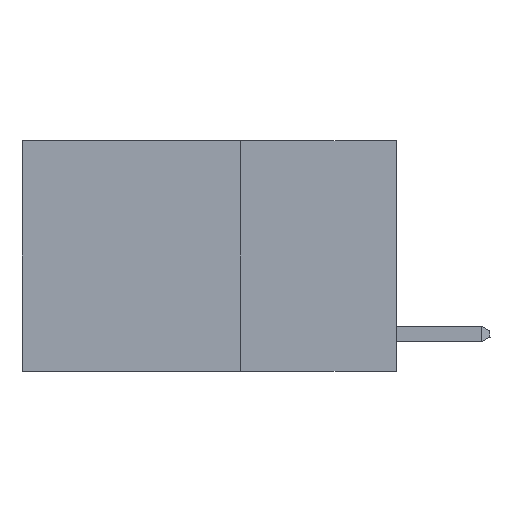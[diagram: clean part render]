
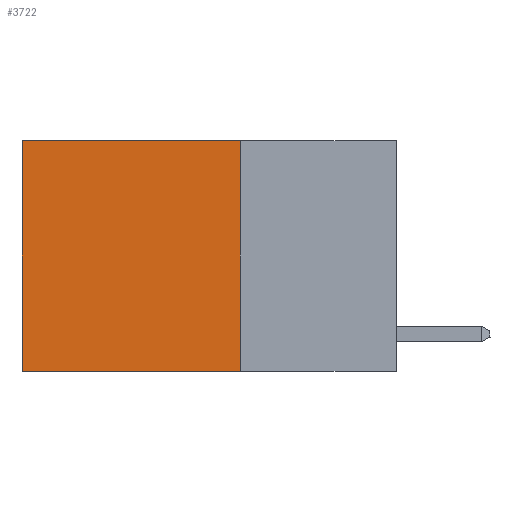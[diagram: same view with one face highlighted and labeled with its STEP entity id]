
A CAD part, left-side view. The second image highlights one B-rep face of the part: STEP entity #3722.
In plain terms, the highlighted planar face has unit normal (-1, 0, 0).
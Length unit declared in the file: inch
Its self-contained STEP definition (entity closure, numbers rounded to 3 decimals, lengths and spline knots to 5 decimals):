
#105 = CARTESIAN_POINT ( 'NONE',  ( 0.2625, 0.6, -0.37 ) ) ;
#321 = CARTESIAN_POINT ( 'NONE',  ( 0.2625, 0.25, -0.37 ) ) ;
#519 = CARTESIAN_POINT ( 'NONE',  ( 0.2625, 0.25, 0. ) ) ;
#686 = DIRECTION ( 'NONE',  ( 0., 0., -1. ) ) ;
#990 = CARTESIAN_POINT ( 'NONE',  ( 0.2625, 0.25, 0. ) ) ;
#2225 = VECTOR ( 'NONE', #8010, 39.37008 ) ;
#2432 = ORIENTED_EDGE ( 'NONE', *, *, #14930, .T. ) ;
#2452 = VERTEX_POINT ( 'NONE', #105 ) ;
#2832 = LINE ( 'NONE', #20732, #2225 ) ;
#3722 = ADVANCED_FACE ( 'NONE', ( #22056 ), #22580, .F. ) ;
#4073 = EDGE_LOOP ( 'NONE', ( #18941, #13759, #9284, #2432 ) ) ;
#4155 = DIRECTION ( 'NONE',  ( 0., 1., 0. ) ) ;
#5664 = VECTOR ( 'NONE', #22316, 39.37008 ) ;
#7095 = EDGE_CURVE ( 'NONE', #8419, #10721, #2832, .T. ) ;
#8010 = DIRECTION ( 'NONE',  ( 0., 0., -1. ) ) ;
#8202 = EDGE_CURVE ( 'NONE', #22284, #2452, #10515, .T. ) ;
#8353 = LINE ( 'NONE', #13313, #17513 ) ;
#8419 = VERTEX_POINT ( 'NONE', #990 ) ;
#9284 = ORIENTED_EDGE ( 'NONE', *, *, #7095, .F. ) ;
#10515 = LINE ( 'NONE', #18725, #5664 ) ;
#10721 = VERTEX_POINT ( 'NONE', #321 ) ;
#10837 = CARTESIAN_POINT ( 'NONE',  ( 0.2625, 0.6, 0. ) ) ;
#11788 = DIRECTION ( 'NONE',  ( 1., 0., 0. ) ) ;
#13313 = CARTESIAN_POINT ( 'NONE',  ( 0.2625, 0.25, 0. ) ) ;
#13759 = ORIENTED_EDGE ( 'NONE', *, *, #17559, .F. ) ;
#14106 = DIRECTION ( 'NONE',  ( 0., 1., 0. ) ) ;
#14930 = EDGE_CURVE ( 'NONE', #8419, #22284, #8353, .T. ) ;
#15381 = VECTOR ( 'NONE', #14106, 39.37008 ) ;
#15956 = LINE ( 'NONE', #23103, #15381 ) ;
#16895 = AXIS2_PLACEMENT_3D ( 'NONE', #519, #11788, #686 ) ;
#17513 = VECTOR ( 'NONE', #4155, 39.37008 ) ;
#17559 = EDGE_CURVE ( 'NONE', #10721, #2452, #15956, .T. ) ;
#18725 = CARTESIAN_POINT ( 'NONE',  ( 0.2625, 0.6, 0. ) ) ;
#18941 = ORIENTED_EDGE ( 'NONE', *, *, #8202, .T. ) ;
#20732 = CARTESIAN_POINT ( 'NONE',  ( 0.2625, 0.25, 0. ) ) ;
#22056 = FACE_OUTER_BOUND ( 'NONE', #4073, .T. ) ;
#22284 = VERTEX_POINT ( 'NONE', #10837 ) ;
#22316 = DIRECTION ( 'NONE',  ( 0., 0., -1. ) ) ;
#22580 = PLANE ( 'NONE',  #16895 ) ;
#23103 = CARTESIAN_POINT ( 'NONE',  ( 0.2625, 0.25, -0.37 ) ) ;
